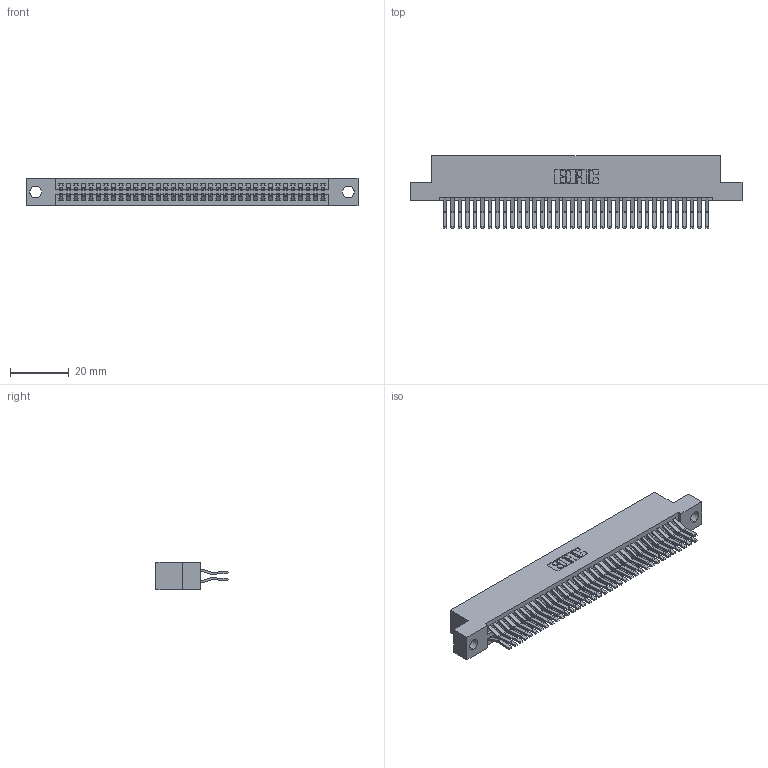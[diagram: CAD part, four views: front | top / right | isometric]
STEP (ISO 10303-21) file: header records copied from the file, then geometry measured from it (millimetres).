
FILE_DESCRIPTION (( 'STEP AP203' ), '1' );
FILE_NAME ('395-072-560-204.STEP', '2018-11-27T16:52:48', ( '' ), ( '' ), 'SwSTEP 2.0', 'SolidWorks 2016', '' );
FILE_SCHEMA (( 'CONFIG_CONTROL_DESIGN' ));
Length unit declared in the file: inch
Products named in the file (3): 345 Part_Flush Mounting Lugs - 0.156 Dia-TH; 345-292-001_560 Tail; 395-072-560-204
Assembly tree (73 placements, depth 2):
  395-072-560-204
    345 Part_Flush Mounting Lugs - 0.156 Dia-TH
    345-292-001_560 Tail  x72
Bounding box: 112.65 x 24.45 x 9.4 mm (x, y, z)
Volume: 11271.2 mm3; surface area: 17573.5 mm2
Topology: 73 solids, 73 shells, 3870 faces, 11501 edges, 7570 vertices
Faces by surface type: plane 2456, cylinder 1414
Entity records: 29145 total; most frequent: CARTESIAN_POINT 4892, ORIENTED_EDGE 4826, DIRECTION 4325, EDGE_CURVE 2413, LINE 2133, VECTOR 2133, VERTEX_POINT 1606, AXIS2_PLACEMENT_3D 1096
